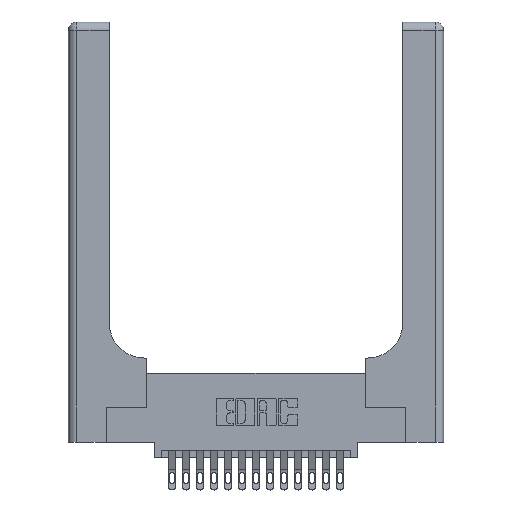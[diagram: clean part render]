
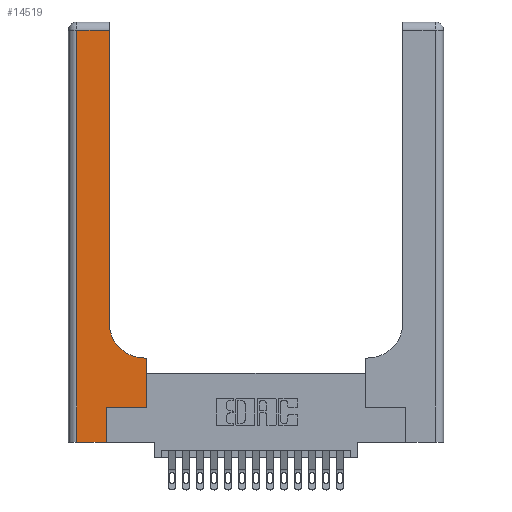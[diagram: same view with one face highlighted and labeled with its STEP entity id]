
A CAD part, top view. The second image highlights one B-rep face of the part: STEP entity #14519.
In plain terms, the highlighted planar face has unit normal (0, 0, 1).
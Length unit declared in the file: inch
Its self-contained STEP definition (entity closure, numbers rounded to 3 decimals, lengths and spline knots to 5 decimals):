
#94 = DIRECTION ( 'NONE',  ( 0., 1., 0. ) ) ;
#398 = LINE ( 'NONE', #2911, #3469 ) ;
#414 = EDGE_CURVE ( 'NONE', #16860, #18341, #5442, .T. ) ;
#713 = CARTESIAN_POINT ( 'NONE',  ( 0., 2.94, 0.37 ) ) ;
#1386 = VECTOR ( 'NONE', #8354, 39.37008 ) ;
#1797 = CARTESIAN_POINT ( 'NONE',  ( 0.5415, 0.6, 0.37 ) ) ;
#1947 = VERTEX_POINT ( 'NONE', #1797 ) ;
#2400 = DIRECTION ( 'NONE',  ( 0., 0., -1. ) ) ;
#2453 = DIRECTION ( 'NONE',  ( 1., 0., 0. ) ) ;
#2605 = CARTESIAN_POINT ( 'NONE',  ( 0.2915, 3., 0.37 ) ) ;
#2911 = CARTESIAN_POINT ( 'NONE',  ( 0.5585, 0.25, 0.37 ) ) ;
#3469 = VECTOR ( 'NONE', #4518, 39.37008 ) ;
#3573 = ORIENTED_EDGE ( 'NONE', *, *, #7601, .T. ) ;
#3926 = ORIENTED_EDGE ( 'NONE', *, *, #9761, .T. ) ;
#4018 = PLANE ( 'NONE',  #7788 ) ;
#4036 = CARTESIAN_POINT ( 'NONE',  ( 0.2915, 2.94, 0.37 ) ) ;
#4425 = CARTESIAN_POINT ( 'NONE',  ( 0.06, 0., 0.37 ) ) ;
#4485 = ORIENTED_EDGE ( 'NONE', *, *, #7829, .T. ) ;
#4518 = DIRECTION ( 'NONE',  ( 0., 1., 0. ) ) ;
#4929 = EDGE_CURVE ( 'NONE', #17292, #6799, #6477, .T. ) ;
#5083 = CIRCLE ( 'NONE', #15996, 0.25 ) ;
#5356 = DIRECTION ( 'NONE',  ( -1., 0., 0. ) ) ;
#5372 = FACE_OUTER_BOUND ( 'NONE', #6081, .T. ) ;
#5442 = LINE ( 'NONE', #713, #1386 ) ;
#5857 = VERTEX_POINT ( 'NONE', #15603 ) ;
#5977 = VERTEX_POINT ( 'NONE', #13961 ) ;
#6081 = EDGE_LOOP ( 'NONE', ( #13215, #13430, #4485, #18895, #3926, #19657, #11517, #16243, #3573 ) ) ;
#6340 = EDGE_CURVE ( 'NONE', #5977, #1947, #11786, .T. ) ;
#6477 = LINE ( 'NONE', #19111, #11217 ) ;
#6799 = VERTEX_POINT ( 'NONE', #8587 ) ;
#7204 = CARTESIAN_POINT ( 'NONE',  ( 0.06, 3., 0.37 ) ) ;
#7601 = EDGE_CURVE ( 'NONE', #1947, #14444, #5083, .T. ) ;
#7788 = AXIS2_PLACEMENT_3D ( 'NONE', #19256, #2400, #5356 ) ;
#7803 = DIRECTION ( 'NONE',  ( 0., 0., -1. ) ) ;
#7829 = EDGE_CURVE ( 'NONE', #18341, #16577, #12942, .T. ) ;
#8354 = DIRECTION ( 'NONE',  ( -1., 0., 0. ) ) ;
#8587 = CARTESIAN_POINT ( 'NONE',  ( 0.5585, 0.25, 0.37 ) ) ;
#8690 = CARTESIAN_POINT ( 'NONE',  ( 0.2915, 0.85, 0.37 ) ) ;
#8719 = DIRECTION ( 'NONE',  ( 0., -1., 0. ) ) ;
#8747 = CARTESIAN_POINT ( 'NONE',  ( 0.06, 2.94, 0.37 ) ) ;
#9049 = LINE ( 'NONE', #2605, #16456 ) ;
#9191 = CARTESIAN_POINT ( 'NONE',  ( 0., 0., 0.37 ) ) ;
#9761 = EDGE_CURVE ( 'NONE', #5857, #17292, #19110, .T. ) ;
#10261 = DIRECTION ( 'NONE',  ( 1., 0., 0. ) ) ;
#11217 = VECTOR ( 'NONE', #2453, 39.37008 ) ;
#11517 = ORIENTED_EDGE ( 'NONE', *, *, #13680, .T. ) ;
#11786 = LINE ( 'NONE', #19260, #13465 ) ;
#11886 = EDGE_CURVE ( 'NONE', #16577, #5857, #19223, .T. ) ;
#12942 = LINE ( 'NONE', #7204, #16291 ) ;
#13215 = ORIENTED_EDGE ( 'NONE', *, *, #18309, .T. ) ;
#13430 = ORIENTED_EDGE ( 'NONE', *, *, #414, .T. ) ;
#13465 = VECTOR ( 'NONE', #16197, 39.37008 ) ;
#13466 = CARTESIAN_POINT ( 'NONE',  ( 0.5415, 0.85, 0.37 ) ) ;
#13680 = EDGE_CURVE ( 'NONE', #6799, #5977, #398, .T. ) ;
#13961 = CARTESIAN_POINT ( 'NONE',  ( 0.5585, 0.6, 0.37 ) ) ;
#14444 = VERTEX_POINT ( 'NONE', #8690 ) ;
#14519 = ADVANCED_FACE ( 'NONE', ( #5372 ), #4018, .F. ) ;
#15452 = VECTOR ( 'NONE', #18856, 39.37008 ) ;
#15603 = CARTESIAN_POINT ( 'NONE',  ( 0.269, 0., 0.37 ) ) ;
#15717 = CARTESIAN_POINT ( 'NONE',  ( 0.269, 0., 0.37 ) ) ;
#15996 = AXIS2_PLACEMENT_3D ( 'NONE', #13466, #7803, #10261 ) ;
#16197 = DIRECTION ( 'NONE',  ( -1., 0., 0. ) ) ;
#16243 = ORIENTED_EDGE ( 'NONE', *, *, #6340, .T. ) ;
#16291 = VECTOR ( 'NONE', #8719, 39.37008 ) ;
#16456 = VECTOR ( 'NONE', #94, 39.37008 ) ;
#16577 = VERTEX_POINT ( 'NONE', #4425 ) ;
#16860 = VERTEX_POINT ( 'NONE', #4036 ) ;
#17292 = VERTEX_POINT ( 'NONE', #18529 ) ;
#18250 = VECTOR ( 'NONE', #18624, 39.37008 ) ;
#18309 = EDGE_CURVE ( 'NONE', #14444, #16860, #9049, .T. ) ;
#18341 = VERTEX_POINT ( 'NONE', #8747 ) ;
#18529 = CARTESIAN_POINT ( 'NONE',  ( 0.269, 0.25, 0.37 ) ) ;
#18624 = DIRECTION ( 'NONE',  ( 1., 0., 0. ) ) ;
#18856 = DIRECTION ( 'NONE',  ( 0., 1., 0. ) ) ;
#18895 = ORIENTED_EDGE ( 'NONE', *, *, #11886, .T. ) ;
#19110 = LINE ( 'NONE', #15717, #15452 ) ;
#19111 = CARTESIAN_POINT ( 'NONE',  ( 0.269, 0.25, 0.37 ) ) ;
#19223 = LINE ( 'NONE', #9191, #18250 ) ;
#19256 = CARTESIAN_POINT ( 'NONE',  ( 0., 3., 0.37 ) ) ;
#19260 = CARTESIAN_POINT ( 'NONE',  ( 0.2915, 0.6, 0.37 ) ) ;
#19657 = ORIENTED_EDGE ( 'NONE', *, *, #4929, .T. ) ;
